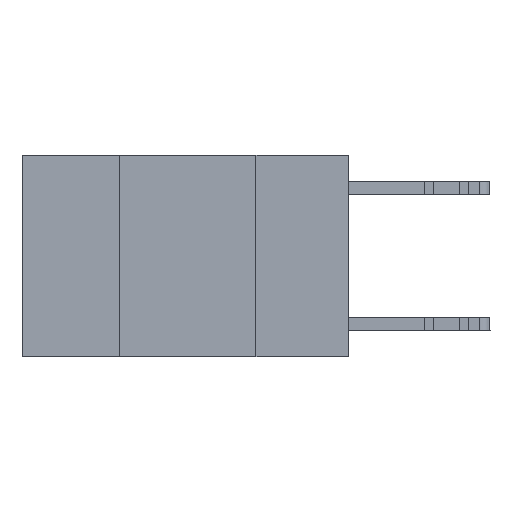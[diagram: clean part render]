
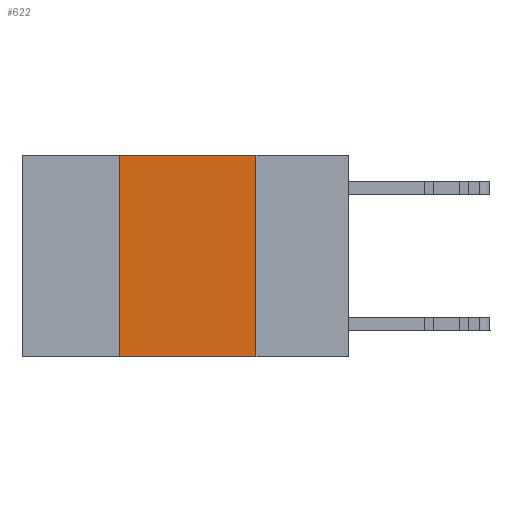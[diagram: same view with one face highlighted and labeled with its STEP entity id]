
A CAD part, left-side view. The second image highlights one B-rep face of the part: STEP entity #622.
In plain terms, the highlighted planar face has unit normal (-1, 0, 0).
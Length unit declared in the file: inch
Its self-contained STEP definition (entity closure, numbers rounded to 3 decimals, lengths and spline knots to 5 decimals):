
#484 = ORIENTED_EDGE ( 'NONE', *, *, #4588, .T. ) ;
#606 = CARTESIAN_POINT ( 'NONE',  ( 0., 0.42, 0. ) ) ;
#622 = ADVANCED_FACE ( 'NONE', ( #28613 ), #11467, .F. ) ;
#1292 = CARTESIAN_POINT ( 'NONE',  ( 0., 0.42, -0.37 ) ) ;
#1343 = VECTOR ( 'NONE', #15208, 39.37008 ) ;
#1481 = LINE ( 'NONE', #26719, #1343 ) ;
#2043 = VECTOR ( 'NONE', #28887, 39.37008 ) ;
#2520 = LINE ( 'NONE', #28605, #2043 ) ;
#2773 = VERTEX_POINT ( 'NONE', #13864 ) ;
#3087 = CARTESIAN_POINT ( 'NONE',  ( 0., 0.17, -0.37 ) ) ;
#3346 = ORIENTED_EDGE ( 'NONE', *, *, #29303, .F. ) ;
#3393 = LINE ( 'NONE', #21613, #3640 ) ;
#3640 = VECTOR ( 'NONE', #21903, 39.37008 ) ;
#4588 = EDGE_CURVE ( 'NONE', #19243, #7949, #3393, .T. ) ;
#7949 = VERTEX_POINT ( 'NONE', #3087 ) ;
#9563 = ORIENTED_EDGE ( 'NONE', *, *, #19134, .F. ) ;
#9567 = EDGE_CURVE ( 'NONE', #2773, #7949, #2520, .T. ) ;
#10591 = EDGE_LOOP ( 'NONE', ( #20214, #9563, #3346, #484 ) ) ;
#10915 = DIRECTION ( 'NONE',  ( 0., 0., -1. ) ) ;
#10956 = DIRECTION ( 'NONE',  ( 1., 0., 0. ) ) ;
#11008 = LINE ( 'NONE', #28048, #22800 ) ;
#11216 = CARTESIAN_POINT ( 'NONE',  ( 0., 0.6, 0. ) ) ;
#11467 = PLANE ( 'NONE',  #18895 ) ;
#13864 = CARTESIAN_POINT ( 'NONE',  ( 0., 0.17, 0. ) ) ;
#14199 = DIRECTION ( 'NONE',  ( 0., 0., 1. ) ) ;
#14333 = VERTEX_POINT ( 'NONE', #606 ) ;
#15208 = DIRECTION ( 'NONE',  ( 0., -1., 0. ) ) ;
#18895 = AXIS2_PLACEMENT_3D ( 'NONE', #11216, #10956, #10915 ) ;
#19134 = EDGE_CURVE ( 'NONE', #14333, #2773, #1481, .T. ) ;
#19243 = VERTEX_POINT ( 'NONE', #1292 ) ;
#20214 = ORIENTED_EDGE ( 'NONE', *, *, #9567, .F. ) ;
#21613 = CARTESIAN_POINT ( 'NONE',  ( 0., 0.6, -0.37 ) ) ;
#21903 = DIRECTION ( 'NONE',  ( 0., -1., 0. ) ) ;
#22800 = VECTOR ( 'NONE', #14199, 39.37008 ) ;
#26719 = CARTESIAN_POINT ( 'NONE',  ( 0., 0.6, 0. ) ) ;
#28048 = CARTESIAN_POINT ( 'NONE',  ( 0., 0.42, 0. ) ) ;
#28605 = CARTESIAN_POINT ( 'NONE',  ( 0., 0.17, 0. ) ) ;
#28613 = FACE_OUTER_BOUND ( 'NONE', #10591, .T. ) ;
#28887 = DIRECTION ( 'NONE',  ( 0., 0., -1. ) ) ;
#29303 = EDGE_CURVE ( 'NONE', #19243, #14333, #11008, .T. ) ;
